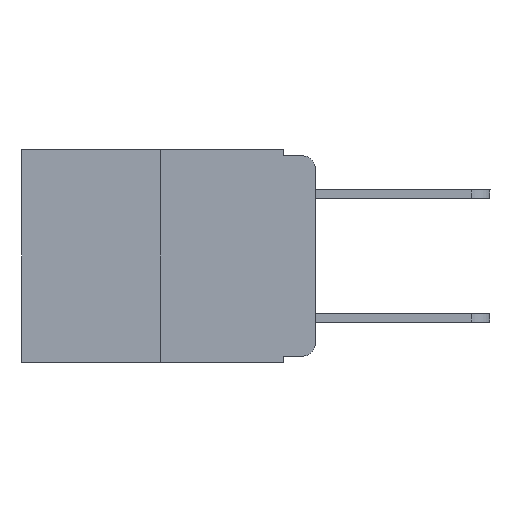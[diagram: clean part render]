
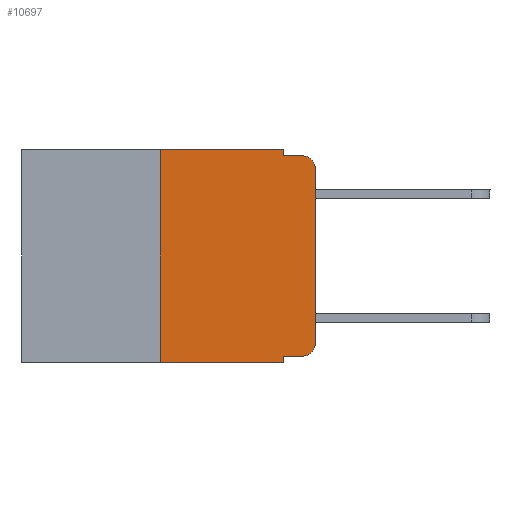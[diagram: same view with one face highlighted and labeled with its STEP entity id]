
A CAD part, left-side view. The second image highlights one B-rep face of the part: STEP entity #10697.
In plain terms, the highlighted planar face has unit normal (-1, 0, 0).
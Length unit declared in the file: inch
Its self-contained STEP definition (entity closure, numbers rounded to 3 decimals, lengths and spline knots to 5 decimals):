
#77 = CARTESIAN_POINT ( 'NONE',  ( 0., 0.051, -0.343 ) ) ;
#195 = AXIS2_PLACEMENT_3D ( 'NONE', #2668, #9848, #5328 ) ;
#411 = EDGE_CURVE ( 'NONE', #4576, #2361, #1466, .T. ) ;
#576 = VECTOR ( 'NONE', #2332, 39.37008 ) ;
#715 = CARTESIAN_POINT ( 'NONE',  ( 0., 0.051, -0.01 ) ) ;
#783 = ORIENTED_EDGE ( 'NONE', *, *, #411, .F. ) ;
#830 = VECTOR ( 'NONE', #11297, 39.37008 ) ;
#1225 = LINE ( 'NONE', #2347, #9354 ) ;
#1466 = LINE ( 'NONE', #8703, #3626 ) ;
#1475 = VECTOR ( 'NONE', #6818, 39.37008 ) ;
#1564 = EDGE_CURVE ( 'NONE', #5565, #2361, #10353, .T. ) ;
#1731 = CIRCLE ( 'NONE', #8381, 0.02 ) ;
#1791 = ORIENTED_EDGE ( 'NONE', *, *, #11092, .T. ) ;
#1994 = LINE ( 'NONE', #3770, #8994 ) ;
#2332 = DIRECTION ( 'NONE',  ( 0., 0., 1. ) ) ;
#2347 = CARTESIAN_POINT ( 'NONE',  ( 0., 0.25, 0. ) ) ;
#2361 = VERTEX_POINT ( 'NONE', #77 ) ;
#2668 = CARTESIAN_POINT ( 'NONE',  ( 0., 0.02, -0.313 ) ) ;
#2901 = DIRECTION ( 'NONE',  ( 0., 0., -1. ) ) ;
#3186 = ORIENTED_EDGE ( 'NONE', *, *, #10740, .T. ) ;
#3491 = ORIENTED_EDGE ( 'NONE', *, *, #1564, .T. ) ;
#3501 = ORIENTED_EDGE ( 'NONE', *, *, #9286, .F. ) ;
#3626 = VECTOR ( 'NONE', #8827, 39.37008 ) ;
#3653 = VECTOR ( 'NONE', #2901, 39.37008 ) ;
#3710 = CARTESIAN_POINT ( 'NONE',  ( 0., 0.02, -0.333 ) ) ;
#3712 = DIRECTION ( 'NONE',  ( 0., -1., 0. ) ) ;
#3770 = CARTESIAN_POINT ( 'NONE',  ( 0., 0.473, 0. ) ) ;
#3840 = CARTESIAN_POINT ( 'NONE',  ( 0., 0.051, -0.01 ) ) ;
#3902 = EDGE_CURVE ( 'NONE', #9690, #10172, #8858, .T. ) ;
#4017 = DIRECTION ( 'NONE',  ( 0., -1., 0. ) ) ;
#4092 = VERTEX_POINT ( 'NONE', #9037 ) ;
#4193 = DIRECTION ( 'NONE',  ( 1., 0., 0. ) ) ;
#4325 = ORIENTED_EDGE ( 'NONE', *, *, #10282, .F. ) ;
#4540 = CARTESIAN_POINT ( 'NONE',  ( 0., 0., -0.03 ) ) ;
#4557 = AXIS2_PLACEMENT_3D ( 'NONE', #6756, #4193, #11381 ) ;
#4576 = VERTEX_POINT ( 'NONE', #9052 ) ;
#4824 = CARTESIAN_POINT ( 'NONE',  ( 0., 0.02, -0.01 ) ) ;
#5328 = DIRECTION ( 'NONE',  ( 0., 0., -1. ) ) ;
#5565 = VERTEX_POINT ( 'NONE', #8538 ) ;
#5599 = CARTESIAN_POINT ( 'NONE',  ( 0., 0.473, -0.343 ) ) ;
#5606 = EDGE_CURVE ( 'NONE', #7034, #4092, #1994, .T. ) ;
#6081 = CARTESIAN_POINT ( 'NONE',  ( 0., 0.25, 0. ) ) ;
#6103 = PLANE ( 'NONE',  #4557 ) ;
#6377 = EDGE_CURVE ( 'NONE', #11318, #9569, #7973, .T. ) ;
#6756 = CARTESIAN_POINT ( 'NONE',  ( 0., 0.473, 0. ) ) ;
#6773 = LINE ( 'NONE', #6832, #576 ) ;
#6818 = DIRECTION ( 'NONE',  ( 0., -1., 0. ) ) ;
#6832 = CARTESIAN_POINT ( 'NONE',  ( 0., 0., 0. ) ) ;
#6909 = ORIENTED_EDGE ( 'NONE', *, *, #5606, .F. ) ;
#7034 = VERTEX_POINT ( 'NONE', #6081 ) ;
#7698 = ORIENTED_EDGE ( 'NONE', *, *, #6377, .T. ) ;
#7729 = EDGE_LOOP ( 'NONE', ( #8568, #3186, #10393, #3501, #6909, #4325, #3491, #783, #1791, #7698 ) ) ;
#7973 = CIRCLE ( 'NONE', #195, 0.02 ) ;
#8077 = CARTESIAN_POINT ( 'NONE',  ( 0., 0.02, -0.03 ) ) ;
#8192 = DIRECTION ( 'NONE',  ( 0., 0., -1. ) ) ;
#8381 = AXIS2_PLACEMENT_3D ( 'NONE', #8077, #9900, #8192 ) ;
#8538 = CARTESIAN_POINT ( 'NONE',  ( 0., 0.25, -0.343 ) ) ;
#8568 = ORIENTED_EDGE ( 'NONE', *, *, #8945, .T. ) ;
#8668 = CARTESIAN_POINT ( 'NONE',  ( 0., 0.051, -0.333 ) ) ;
#8703 = CARTESIAN_POINT ( 'NONE',  ( 0., 0.051, 0. ) ) ;
#8779 = VECTOR ( 'NONE', #4017, 39.37008 ) ;
#8827 = DIRECTION ( 'NONE',  ( 0., 0., -1. ) ) ;
#8857 = FACE_OUTER_BOUND ( 'NONE', #7729, .T. ) ;
#8858 = LINE ( 'NONE', #715, #1475 ) ;
#8945 = EDGE_CURVE ( 'NONE', #9569, #9457, #6773, .T. ) ;
#8994 = VECTOR ( 'NONE', #3712, 39.37008 ) ;
#9037 = CARTESIAN_POINT ( 'NONE',  ( 0., 0.051, 0. ) ) ;
#9052 = CARTESIAN_POINT ( 'NONE',  ( 0., 0.051, -0.333 ) ) ;
#9286 = EDGE_CURVE ( 'NONE', #4092, #9690, #11028, .T. ) ;
#9354 = VECTOR ( 'NONE', #10354, 39.37008 ) ;
#9457 = VERTEX_POINT ( 'NONE', #4540 ) ;
#9569 = VERTEX_POINT ( 'NONE', #9726 ) ;
#9605 = LINE ( 'NONE', #8668, #8779 ) ;
#9690 = VERTEX_POINT ( 'NONE', #3840 ) ;
#9726 = CARTESIAN_POINT ( 'NONE',  ( 0., 0., -0.313 ) ) ;
#9848 = DIRECTION ( 'NONE',  ( -1., 0., 0. ) ) ;
#9900 = DIRECTION ( 'NONE',  ( -1., 0., 0. ) ) ;
#10172 = VERTEX_POINT ( 'NONE', #4824 ) ;
#10282 = EDGE_CURVE ( 'NONE', #5565, #7034, #1225, .T. ) ;
#10353 = LINE ( 'NONE', #5599, #830 ) ;
#10354 = DIRECTION ( 'NONE',  ( 0., 0., 1. ) ) ;
#10393 = ORIENTED_EDGE ( 'NONE', *, *, #3902, .F. ) ;
#10697 = ADVANCED_FACE ( 'NONE', ( #8857 ), #6103, .F. ) ;
#10740 = EDGE_CURVE ( 'NONE', #9457, #10172, #1731, .T. ) ;
#11028 = LINE ( 'NONE', #11088, #3653 ) ;
#11088 = CARTESIAN_POINT ( 'NONE',  ( 0., 0.051, 0. ) ) ;
#11092 = EDGE_CURVE ( 'NONE', #4576, #11318, #9605, .T. ) ;
#11297 = DIRECTION ( 'NONE',  ( 0., -1., 0. ) ) ;
#11318 = VERTEX_POINT ( 'NONE', #3710 ) ;
#11381 = DIRECTION ( 'NONE',  ( 0., 0., -1. ) ) ;
